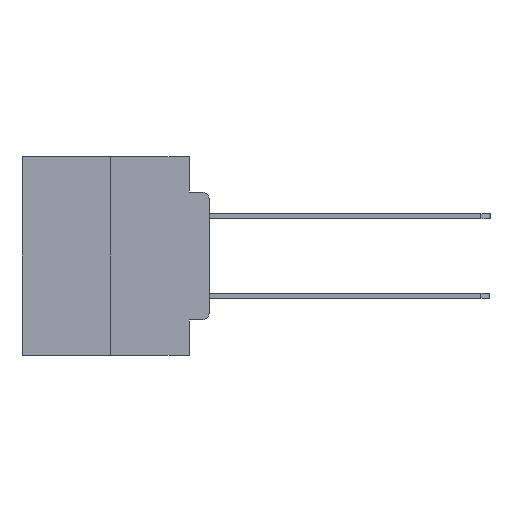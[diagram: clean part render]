
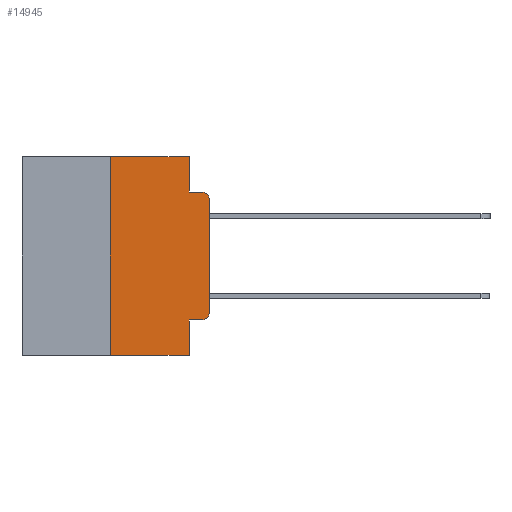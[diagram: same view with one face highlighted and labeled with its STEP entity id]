
A CAD part, left-side view. The second image highlights one B-rep face of the part: STEP entity #14945.
In plain terms, the highlighted planar face has unit normal (-1, 0, 0).
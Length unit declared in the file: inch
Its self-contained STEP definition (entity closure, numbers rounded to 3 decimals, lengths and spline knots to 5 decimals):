
#199 = CARTESIAN_POINT ( 'NONE',  ( 0., 0.25, -0.5 ) ) ;
#1171 = CARTESIAN_POINT ( 'NONE',  ( 0., 0.02, -0.3915 ) ) ;
#1677 = DIRECTION ( 'NONE',  ( 0., -1., 0. ) ) ;
#2330 = EDGE_CURVE ( 'NONE', #21733, #11745, #22393, .T. ) ;
#2334 = ORIENTED_EDGE ( 'NONE', *, *, #15415, .T. ) ;
#2626 = DIRECTION ( 'NONE',  ( 0., 0., 1. ) ) ;
#3075 = LINE ( 'NONE', #9422, #10648 ) ;
#3130 = PLANE ( 'NONE',  #13789 ) ;
#3362 = DIRECTION ( 'NONE',  ( 0., 0., -1. ) ) ;
#3641 = CARTESIAN_POINT ( 'NONE',  ( 0., 0.25, 0. ) ) ;
#3789 = ORIENTED_EDGE ( 'NONE', *, *, #26156, .T. ) ;
#4147 = CARTESIAN_POINT ( 'NONE',  ( 0., 0.051, 0. ) ) ;
#4184 = CARTESIAN_POINT ( 'NONE',  ( 0., 0.051, -0.0885 ) ) ;
#5555 = VECTOR ( 'NONE', #9928, 39.37008 ) ;
#5679 = CARTESIAN_POINT ( 'NONE',  ( 0., 0.051, -0.4115 ) ) ;
#6217 = ORIENTED_EDGE ( 'NONE', *, *, #7193, .F. ) ;
#6512 = EDGE_LOOP ( 'NONE', ( #6830, #3789, #15670, #22699, #6217, #20160, #21513, #17226, #15551, #2334 ) ) ;
#6566 = VECTOR ( 'NONE', #21089, 39.37008 ) ;
#6830 = ORIENTED_EDGE ( 'NONE', *, *, #2330, .T. ) ;
#7143 = CARTESIAN_POINT ( 'NONE',  ( 0., 0.051, -0.5 ) ) ;
#7193 = EDGE_CURVE ( 'NONE', #15506, #11469, #25324, .T. ) ;
#7224 = VECTOR ( 'NONE', #24658, 39.37008 ) ;
#7406 = DIRECTION ( 'NONE',  ( 0., 0., -1. ) ) ;
#7882 = CARTESIAN_POINT ( 'NONE',  ( 0., 0.473, 0. ) ) ;
#7959 = CARTESIAN_POINT ( 'NONE',  ( 0., 0.051, -0.0885 ) ) ;
#8304 = VERTEX_POINT ( 'NONE', #5679 ) ;
#8952 = CARTESIAN_POINT ( 'NONE',  ( 0., 0.02, -0.0885 ) ) ;
#9206 = EDGE_CURVE ( 'NONE', #15783, #15506, #23604, .T. ) ;
#9422 = CARTESIAN_POINT ( 'NONE',  ( 0., 0.473, -0.5 ) ) ;
#9840 = CARTESIAN_POINT ( 'NONE',  ( 0., 0., 0. ) ) ;
#9928 = DIRECTION ( 'NONE',  ( 0., 0., 1. ) ) ;
#9979 = EDGE_CURVE ( 'NONE', #15783, #13695, #3075, .T. ) ;
#10613 = EDGE_CURVE ( 'NONE', #11469, #19023, #13496, .T. ) ;
#10648 = VECTOR ( 'NONE', #22108, 39.37008 ) ;
#11125 = AXIS2_PLACEMENT_3D ( 'NONE', #11387, #26119, #13515 ) ;
#11387 = CARTESIAN_POINT ( 'NONE',  ( 0., 0.02, -0.1085 ) ) ;
#11469 = VERTEX_POINT ( 'NONE', #20163 ) ;
#11745 = VERTEX_POINT ( 'NONE', #17293 ) ;
#12352 = VECTOR ( 'NONE', #2626, 39.37008 ) ;
#12495 = CIRCLE ( 'NONE', #21765, 0.02 ) ;
#12587 = DIRECTION ( 'NONE',  ( 0., 0., -1. ) ) ;
#13411 = VERTEX_POINT ( 'NONE', #27186 ) ;
#13496 = LINE ( 'NONE', #26328, #24719 ) ;
#13515 = DIRECTION ( 'NONE',  ( 0., 0., -1. ) ) ;
#13695 = VERTEX_POINT ( 'NONE', #7143 ) ;
#13738 = DIRECTION ( 'NONE',  ( 0., 0., -1. ) ) ;
#13789 = AXIS2_PLACEMENT_3D ( 'NONE', #17930, #20053, #7406 ) ;
#14945 = ADVANCED_FACE ( 'NONE', ( #23122 ), #3130, .F. ) ;
#15415 = EDGE_CURVE ( 'NONE', #13411, #21733, #12495, .T. ) ;
#15506 = VERTEX_POINT ( 'NONE', #3641 ) ;
#15551 = ORIENTED_EDGE ( 'NONE', *, *, #16863, .T. ) ;
#15670 = ORIENTED_EDGE ( 'NONE', *, *, #19155, .F. ) ;
#15783 = VERTEX_POINT ( 'NONE', #199 ) ;
#16012 = DIRECTION ( 'NONE',  ( -1., 0., 0. ) ) ;
#16863 = EDGE_CURVE ( 'NONE', #8304, #13411, #24812, .T. ) ;
#17226 = ORIENTED_EDGE ( 'NONE', *, *, #22509, .F. ) ;
#17293 = CARTESIAN_POINT ( 'NONE',  ( 0., 0., -0.1085 ) ) ;
#17700 = VERTEX_POINT ( 'NONE', #8952 ) ;
#17930 = CARTESIAN_POINT ( 'NONE',  ( 0., 0.473, 0. ) ) ;
#18587 = VECTOR ( 'NONE', #1677, 39.37008 ) ;
#19023 = VERTEX_POINT ( 'NONE', #7959 ) ;
#19155 = EDGE_CURVE ( 'NONE', #19023, #17700, #24041, .T. ) ;
#19557 = CARTESIAN_POINT ( 'NONE',  ( 0., 0.25, 0. ) ) ;
#19626 = VECTOR ( 'NONE', #12587, 39.37008 ) ;
#20053 = DIRECTION ( 'NONE',  ( 1., 0., 0. ) ) ;
#20160 = ORIENTED_EDGE ( 'NONE', *, *, #9206, .F. ) ;
#20163 = CARTESIAN_POINT ( 'NONE',  ( 0., 0.051, 0. ) ) ;
#21089 = DIRECTION ( 'NONE',  ( 0., -1., 0. ) ) ;
#21513 = ORIENTED_EDGE ( 'NONE', *, *, #9979, .T. ) ;
#21733 = VERTEX_POINT ( 'NONE', #22641 ) ;
#21765 = AXIS2_PLACEMENT_3D ( 'NONE', #1171, #16012, #3362 ) ;
#22108 = DIRECTION ( 'NONE',  ( 0., -1., 0. ) ) ;
#22393 = LINE ( 'NONE', #9840, #5555 ) ;
#22509 = EDGE_CURVE ( 'NONE', #8304, #13695, #25187, .T. ) ;
#22641 = CARTESIAN_POINT ( 'NONE',  ( 0., 0., -0.3915 ) ) ;
#22699 = ORIENTED_EDGE ( 'NONE', *, *, #10613, .F. ) ;
#23122 = FACE_OUTER_BOUND ( 'NONE', #6512, .T. ) ;
#23604 = LINE ( 'NONE', #19557, #12352 ) ;
#24041 = LINE ( 'NONE', #4184, #6566 ) ;
#24658 = DIRECTION ( 'NONE',  ( 0., -1., 0. ) ) ;
#24719 = VECTOR ( 'NONE', #13738, 39.37008 ) ;
#24812 = LINE ( 'NONE', #26932, #18587 ) ;
#25187 = LINE ( 'NONE', #4147, #19626 ) ;
#25324 = LINE ( 'NONE', #7882, #7224 ) ;
#25499 = CIRCLE ( 'NONE', #11125, 0.02 ) ;
#26119 = DIRECTION ( 'NONE',  ( -1., 0., 0. ) ) ;
#26156 = EDGE_CURVE ( 'NONE', #11745, #17700, #25499, .T. ) ;
#26328 = CARTESIAN_POINT ( 'NONE',  ( 0., 0.051, 0. ) ) ;
#26932 = CARTESIAN_POINT ( 'NONE',  ( 0., 0.051, -0.4115 ) ) ;
#27186 = CARTESIAN_POINT ( 'NONE',  ( 0., 0.02, -0.4115 ) ) ;
